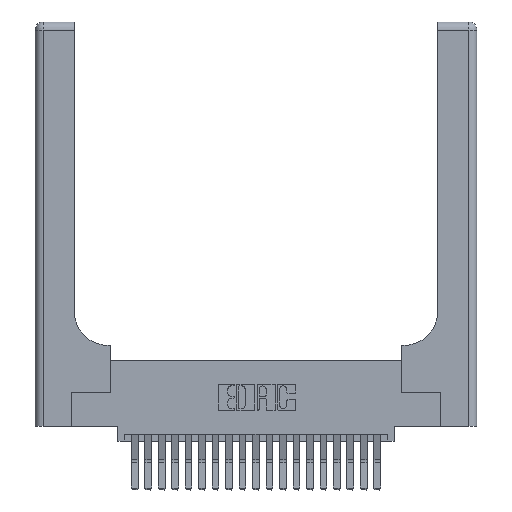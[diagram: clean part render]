
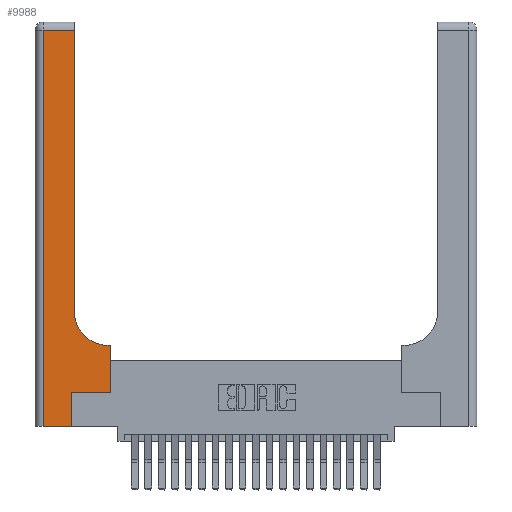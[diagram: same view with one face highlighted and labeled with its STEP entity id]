
A CAD part, top view. The second image highlights one B-rep face of the part: STEP entity #9988.
In plain terms, the highlighted planar face has unit normal (0, 0, 1).
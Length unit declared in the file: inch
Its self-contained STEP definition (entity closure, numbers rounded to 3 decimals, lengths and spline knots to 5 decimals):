
#123 = EDGE_LOOP ( 'NONE', ( #2819, #1015, #12791, #18427, #1205, #15926, #5961, #8543, #7398 ) ) ;
#452 = EDGE_CURVE ( 'NONE', #2474, #10629, #20283, .T. ) ;
#1015 = ORIENTED_EDGE ( 'NONE', *, *, #21532, .T. ) ;
#1205 = ORIENTED_EDGE ( 'NONE', *, *, #21438, .T. ) ;
#1802 = VECTOR ( 'NONE', #10392, 39.37008 ) ;
#1862 = VERTEX_POINT ( 'NONE', #6799 ) ;
#2041 = LINE ( 'NONE', #17805, #16075 ) ;
#2227 = VERTEX_POINT ( 'NONE', #13692 ) ;
#2474 = VERTEX_POINT ( 'NONE', #14132 ) ;
#2819 = ORIENTED_EDGE ( 'NONE', *, *, #11360, .T. ) ;
#3109 = DIRECTION ( 'NONE',  ( 0., 1., 0. ) ) ;
#3636 = CARTESIAN_POINT ( 'NONE',  ( 0.5415, 0.85, 0.37 ) ) ;
#5060 = EDGE_CURVE ( 'NONE', #7712, #1862, #2041, .T. ) ;
#5149 = DIRECTION ( 'NONE',  ( -1., 0., 0. ) ) ;
#5479 = CARTESIAN_POINT ( 'NONE',  ( 0.5585, 0.25, 0.37 ) ) ;
#5499 = DIRECTION ( 'NONE',  ( 1., 0., 0. ) ) ;
#5653 = DIRECTION ( 'NONE',  ( 0., 1., 0. ) ) ;
#5924 = VECTOR ( 'NONE', #11964, 39.37008 ) ;
#5961 = ORIENTED_EDGE ( 'NONE', *, *, #18246, .T. ) ;
#6220 = CARTESIAN_POINT ( 'NONE',  ( 0.269, 0.25, 0.37 ) ) ;
#6327 = AXIS2_PLACEMENT_3D ( 'NONE', #10541, #16030, #5149 ) ;
#6507 = VERTEX_POINT ( 'NONE', #9705 ) ;
#6776 = CARTESIAN_POINT ( 'NONE',  ( 0.2915, 0.6, 0.37 ) ) ;
#6799 = CARTESIAN_POINT ( 'NONE',  ( 0.269, 0., 0.37 ) ) ;
#6897 = DIRECTION ( 'NONE',  ( 0., -1., 0. ) ) ;
#7398 = ORIENTED_EDGE ( 'NONE', *, *, #10798, .T. ) ;
#7712 = VERTEX_POINT ( 'NONE', #11153 ) ;
#7792 = VECTOR ( 'NONE', #6897, 39.37008 ) ;
#8543 = ORIENTED_EDGE ( 'NONE', *, *, #452, .T. ) ;
#8636 = VECTOR ( 'NONE', #5653, 39.37008 ) ;
#8928 = LINE ( 'NONE', #22865, #7792 ) ;
#9044 = VECTOR ( 'NONE', #11979, 39.37008 ) ;
#9235 = VECTOR ( 'NONE', #20592, 39.37008 ) ;
#9705 = CARTESIAN_POINT ( 'NONE',  ( 0.269, 0.25, 0.37 ) ) ;
#9988 = ADVANCED_FACE ( 'NONE', ( #19750 ), #15952, .F. ) ;
#10392 = DIRECTION ( 'NONE',  ( -1., 0., 0. ) ) ;
#10541 = CARTESIAN_POINT ( 'NONE',  ( 0., 3., 0.37 ) ) ;
#10629 = VERTEX_POINT ( 'NONE', #12257 ) ;
#10798 = EDGE_CURVE ( 'NONE', #10629, #12038, #19384, .T. ) ;
#11153 = CARTESIAN_POINT ( 'NONE',  ( 0.06, 0., 0.37 ) ) ;
#11360 = EDGE_CURVE ( 'NONE', #12038, #23345, #17694, .T. ) ;
#11964 = DIRECTION ( 'NONE',  ( -1., 0., 0. ) ) ;
#11979 = DIRECTION ( 'NONE',  ( 0., 1., 0. ) ) ;
#12038 = VERTEX_POINT ( 'NONE', #12414 ) ;
#12257 = CARTESIAN_POINT ( 'NONE',  ( 0.5415, 0.6, 0.37 ) ) ;
#12414 = CARTESIAN_POINT ( 'NONE',  ( 0.2915, 0.85, 0.37 ) ) ;
#12791 = ORIENTED_EDGE ( 'NONE', *, *, #18038, .T. ) ;
#12878 = VECTOR ( 'NONE', #3109, 39.37008 ) ;
#13256 = LINE ( 'NONE', #20874, #9044 ) ;
#13692 = CARTESIAN_POINT ( 'NONE',  ( 0.06, 2.94, 0.37 ) ) ;
#14028 = CARTESIAN_POINT ( 'NONE',  ( 0., 2.94, 0.37 ) ) ;
#14132 = CARTESIAN_POINT ( 'NONE',  ( 0.5585, 0.6, 0.37 ) ) ;
#14702 = CARTESIAN_POINT ( 'NONE',  ( 0.5585, 0.25, 0.37 ) ) ;
#14970 = VERTEX_POINT ( 'NONE', #5479 ) ;
#15154 = AXIS2_PLACEMENT_3D ( 'NONE', #3636, #16377, #5499 ) ;
#15809 = CARTESIAN_POINT ( 'NONE',  ( 0.2915, 3., 0.37 ) ) ;
#15926 = ORIENTED_EDGE ( 'NONE', *, *, #16728, .T. ) ;
#15952 = PLANE ( 'NONE',  #6327 ) ;
#16030 = DIRECTION ( 'NONE',  ( 0., 0., -1. ) ) ;
#16075 = VECTOR ( 'NONE', #19585, 39.37008 ) ;
#16377 = DIRECTION ( 'NONE',  ( 0., 0., -1. ) ) ;
#16399 = LINE ( 'NONE', #14028, #1802 ) ;
#16728 = EDGE_CURVE ( 'NONE', #6507, #14970, #18253, .T. ) ;
#17694 = LINE ( 'NONE', #15809, #12878 ) ;
#17805 = CARTESIAN_POINT ( 'NONE',  ( 0., 0., 0.37 ) ) ;
#18038 = EDGE_CURVE ( 'NONE', #2227, #7712, #8928, .T. ) ;
#18210 = LINE ( 'NONE', #14702, #8636 ) ;
#18246 = EDGE_CURVE ( 'NONE', #14970, #2474, #18210, .T. ) ;
#18253 = LINE ( 'NONE', #6220, #9235 ) ;
#18427 = ORIENTED_EDGE ( 'NONE', *, *, #5060, .T. ) ;
#19384 = CIRCLE ( 'NONE', #15154, 0.25 ) ;
#19585 = DIRECTION ( 'NONE',  ( 1., 0., 0. ) ) ;
#19750 = FACE_OUTER_BOUND ( 'NONE', #123, .T. ) ;
#20283 = LINE ( 'NONE', #6776, #5924 ) ;
#20592 = DIRECTION ( 'NONE',  ( 1., 0., 0. ) ) ;
#20799 = CARTESIAN_POINT ( 'NONE',  ( 0.2915, 2.94, 0.37 ) ) ;
#20874 = CARTESIAN_POINT ( 'NONE',  ( 0.269, 0., 0.37 ) ) ;
#21438 = EDGE_CURVE ( 'NONE', #1862, #6507, #13256, .T. ) ;
#21532 = EDGE_CURVE ( 'NONE', #23345, #2227, #16399, .T. ) ;
#22865 = CARTESIAN_POINT ( 'NONE',  ( 0.06, 3., 0.37 ) ) ;
#23345 = VERTEX_POINT ( 'NONE', #20799 ) ;
